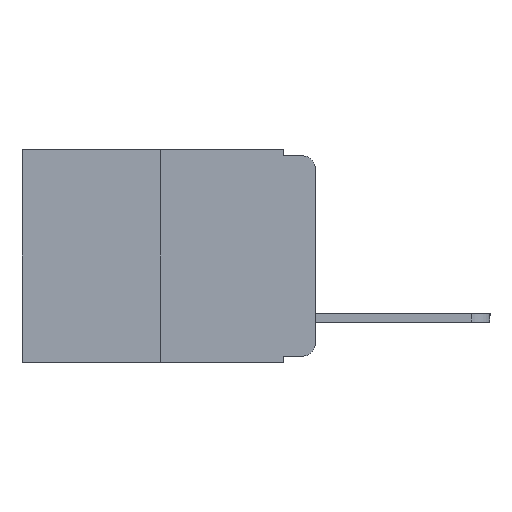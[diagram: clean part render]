
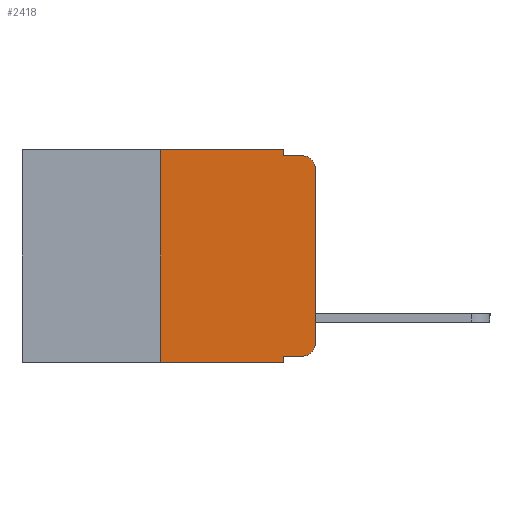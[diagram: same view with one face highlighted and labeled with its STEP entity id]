
A CAD part, left-side view. The second image highlights one B-rep face of the part: STEP entity #2418.
In plain terms, the highlighted planar face has unit normal (-1, 0, 0).
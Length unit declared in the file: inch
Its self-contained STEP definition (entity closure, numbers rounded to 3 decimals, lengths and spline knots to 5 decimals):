
#74 = ORIENTED_EDGE ( 'NONE', *, *, #8228, .F. ) ;
#277 = VERTEX_POINT ( 'NONE', #732 ) ;
#475 = AXIS2_PLACEMENT_3D ( 'NONE', #10800, #10783, #10094 ) ;
#572 = LINE ( 'NONE', #1244, #9174 ) ;
#591 = CARTESIAN_POINT ( 'NONE',  ( 0., 0.051, -0.01 ) ) ;
#695 = CARTESIAN_POINT ( 'NONE',  ( 0., 0.473, 0. ) ) ;
#732 = CARTESIAN_POINT ( 'NONE',  ( 0., 0., -0.03 ) ) ;
#791 = VERTEX_POINT ( 'NONE', #1052 ) ;
#915 = VERTEX_POINT ( 'NONE', #5061 ) ;
#917 = AXIS2_PLACEMENT_3D ( 'NONE', #7695, #8559, #9533 ) ;
#1052 = CARTESIAN_POINT ( 'NONE',  ( 0., 0.25, 0. ) ) ;
#1068 = VECTOR ( 'NONE', #4974, 39.37008 ) ;
#1244 = CARTESIAN_POINT ( 'NONE',  ( 0., 0.051, -0.01 ) ) ;
#1301 = EDGE_CURVE ( 'NONE', #10033, #4013, #1573, .T. ) ;
#1573 = LINE ( 'NONE', #5939, #10466 ) ;
#1656 = EDGE_CURVE ( 'NONE', #5538, #2013, #9850, .T. ) ;
#1707 = VERTEX_POINT ( 'NONE', #7588 ) ;
#1823 = CIRCLE ( 'NONE', #475, 0.02 ) ;
#1829 = EDGE_LOOP ( 'NONE', ( #10646, #6160, #74, #2359, #10001, #7639, #10018, #6864, #1981, #7527 ) ) ;
#1981 = ORIENTED_EDGE ( 'NONE', *, *, #9955, .T. ) ;
#2001 = PLANE ( 'NONE',  #8094 ) ;
#2013 = VERTEX_POINT ( 'NONE', #591 ) ;
#2147 = CARTESIAN_POINT ( 'NONE',  ( 0., 0.02, -0.01 ) ) ;
#2359 = ORIENTED_EDGE ( 'NONE', *, *, #1656, .F. ) ;
#2418 = ADVANCED_FACE ( 'NONE', ( #10320 ), #2001, .F. ) ;
#2579 = VECTOR ( 'NONE', #5392, 39.37008 ) ;
#2763 = EDGE_CURVE ( 'NONE', #10033, #791, #7317, .T. ) ;
#2839 = CARTESIAN_POINT ( 'NONE',  ( 0., 0.051, -0.343 ) ) ;
#2925 = EDGE_CURVE ( 'NONE', #4892, #277, #5683, .T. ) ;
#3134 = DIRECTION ( 'NONE',  ( 0., 0., -1. ) ) ;
#3323 = CARTESIAN_POINT ( 'NONE',  ( 0., 0.051, -0.333 ) ) ;
#3377 = CARTESIAN_POINT ( 'NONE',  ( 0., 0., -0.313 ) ) ;
#3471 = CARTESIAN_POINT ( 'NONE',  ( 0., 0.473, 0. ) ) ;
#4013 = VERTEX_POINT ( 'NONE', #2839 ) ;
#4091 = VERTEX_POINT ( 'NONE', #2147 ) ;
#4133 = EDGE_CURVE ( 'NONE', #1707, #4013, #5956, .T. ) ;
#4331 = EDGE_CURVE ( 'NONE', #915, #4892, #1823, .T. ) ;
#4514 = CARTESIAN_POINT ( 'NONE',  ( 0., 0.25, 0. ) ) ;
#4892 = VERTEX_POINT ( 'NONE', #3377 ) ;
#4974 = DIRECTION ( 'NONE',  ( 0., 0., 1. ) ) ;
#5061 = CARTESIAN_POINT ( 'NONE',  ( 0., 0.02, -0.333 ) ) ;
#5392 = DIRECTION ( 'NONE',  ( 0., 0., 1. ) ) ;
#5448 = VECTOR ( 'NONE', #5684, 39.37008 ) ;
#5538 = VERTEX_POINT ( 'NONE', #6632 ) ;
#5683 = LINE ( 'NONE', #7447, #1068 ) ;
#5684 = DIRECTION ( 'NONE',  ( 0., 0., -1. ) ) ;
#5939 = CARTESIAN_POINT ( 'NONE',  ( 0., 0.473, -0.343 ) ) ;
#5956 = LINE ( 'NONE', #11038, #8202 ) ;
#6160 = ORIENTED_EDGE ( 'NONE', *, *, #9028, .T. ) ;
#6632 = CARTESIAN_POINT ( 'NONE',  ( 0., 0.051, 0. ) ) ;
#6692 = DIRECTION ( 'NONE',  ( 0., -1., 0. ) ) ;
#6864 = ORIENTED_EDGE ( 'NONE', *, *, #4133, .F. ) ;
#6866 = LINE ( 'NONE', #3323, #8766 ) ;
#7317 = LINE ( 'NONE', #4514, #2579 ) ;
#7447 = CARTESIAN_POINT ( 'NONE',  ( 0., 0., 0. ) ) ;
#7527 = ORIENTED_EDGE ( 'NONE', *, *, #4331, .T. ) ;
#7588 = CARTESIAN_POINT ( 'NONE',  ( 0., 0.051, -0.333 ) ) ;
#7639 = ORIENTED_EDGE ( 'NONE', *, *, #2763, .F. ) ;
#7695 = CARTESIAN_POINT ( 'NONE',  ( 0., 0.02, -0.03 ) ) ;
#7919 = DIRECTION ( 'NONE',  ( 0., -1., 0. ) ) ;
#7962 = DIRECTION ( 'NONE',  ( 0., 0., -1. ) ) ;
#8094 = AXIS2_PLACEMENT_3D ( 'NONE', #3471, #8649, #7962 ) ;
#8202 = VECTOR ( 'NONE', #3134, 39.37008 ) ;
#8228 = EDGE_CURVE ( 'NONE', #2013, #4091, #572, .T. ) ;
#8402 = DIRECTION ( 'NONE',  ( 0., -1., 0. ) ) ;
#8498 = CARTESIAN_POINT ( 'NONE',  ( 0., 0.051, 0. ) ) ;
#8559 = DIRECTION ( 'NONE',  ( -1., 0., 0. ) ) ;
#8649 = DIRECTION ( 'NONE',  ( 1., 0., 0. ) ) ;
#8664 = EDGE_CURVE ( 'NONE', #791, #5538, #8913, .T. ) ;
#8766 = VECTOR ( 'NONE', #10860, 39.37008 ) ;
#8913 = LINE ( 'NONE', #695, #10775 ) ;
#9028 = EDGE_CURVE ( 'NONE', #277, #4091, #9153, .T. ) ;
#9153 = CIRCLE ( 'NONE', #917, 0.02 ) ;
#9174 = VECTOR ( 'NONE', #6692, 39.37008 ) ;
#9533 = DIRECTION ( 'NONE',  ( 0., 0., -1. ) ) ;
#9850 = LINE ( 'NONE', #8498, #5448 ) ;
#9955 = EDGE_CURVE ( 'NONE', #1707, #915, #6866, .T. ) ;
#10001 = ORIENTED_EDGE ( 'NONE', *, *, #8664, .F. ) ;
#10018 = ORIENTED_EDGE ( 'NONE', *, *, #1301, .T. ) ;
#10023 = CARTESIAN_POINT ( 'NONE',  ( 0., 0.25, -0.343 ) ) ;
#10033 = VERTEX_POINT ( 'NONE', #10023 ) ;
#10094 = DIRECTION ( 'NONE',  ( 0., 0., -1. ) ) ;
#10320 = FACE_OUTER_BOUND ( 'NONE', #1829, .T. ) ;
#10466 = VECTOR ( 'NONE', #8402, 39.37008 ) ;
#10646 = ORIENTED_EDGE ( 'NONE', *, *, #2925, .T. ) ;
#10775 = VECTOR ( 'NONE', #7919, 39.37008 ) ;
#10783 = DIRECTION ( 'NONE',  ( -1., 0., 0. ) ) ;
#10800 = CARTESIAN_POINT ( 'NONE',  ( 0., 0.02, -0.313 ) ) ;
#10860 = DIRECTION ( 'NONE',  ( 0., -1., 0. ) ) ;
#11038 = CARTESIAN_POINT ( 'NONE',  ( 0., 0.051, 0. ) ) ;
